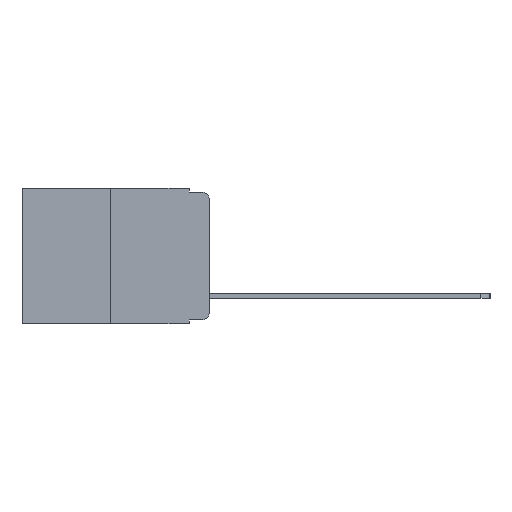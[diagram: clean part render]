
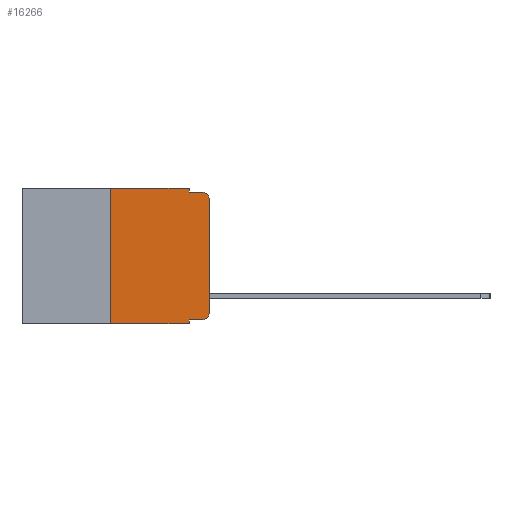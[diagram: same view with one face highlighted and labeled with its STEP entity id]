
A CAD part, left-side view. The second image highlights one B-rep face of the part: STEP entity #16266.
In plain terms, the highlighted planar face has unit normal (-1, 0, 0).
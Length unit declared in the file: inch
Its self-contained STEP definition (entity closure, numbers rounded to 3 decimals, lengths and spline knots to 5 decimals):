
#207 = CARTESIAN_POINT ( 'NONE',  ( 0., 0.051, -0.333 ) ) ;
#868 = ORIENTED_EDGE ( 'NONE', *, *, #16765, .T. ) ;
#1029 = DIRECTION ( 'NONE',  ( -1., 0., 0. ) ) ;
#1169 = CARTESIAN_POINT ( 'NONE',  ( 0., 0., -0.03 ) ) ;
#1591 = VECTOR ( 'NONE', #9328, 39.37008 ) ;
#1666 = VERTEX_POINT ( 'NONE', #6578 ) ;
#1688 = ORIENTED_EDGE ( 'NONE', *, *, #2885, .T. ) ;
#2386 = LINE ( 'NONE', #5557, #13495 ) ;
#2468 = EDGE_LOOP ( 'NONE', ( #868, #10151, #3835, #2747, #3150, #14871, #12457, #14126, #10528, #1688 ) ) ;
#2552 = DIRECTION ( 'NONE',  ( 0., -1., 0. ) ) ;
#2593 = CARTESIAN_POINT ( 'NONE',  ( 0., 0.051, 0. ) ) ;
#2747 = ORIENTED_EDGE ( 'NONE', *, *, #11680, .F. ) ;
#2823 = CIRCLE ( 'NONE', #15723, 0.02 ) ;
#2885 = EDGE_CURVE ( 'NONE', #5201, #4360, #8618, .T. ) ;
#2953 = VERTEX_POINT ( 'NONE', #6489 ) ;
#3044 = AXIS2_PLACEMENT_3D ( 'NONE', #14238, #14297, #5747 ) ;
#3091 = DIRECTION ( 'NONE',  ( 0., 0., -1. ) ) ;
#3150 = ORIENTED_EDGE ( 'NONE', *, *, #5039, .F. ) ;
#3338 = LINE ( 'NONE', #12954, #6807 ) ;
#3835 = ORIENTED_EDGE ( 'NONE', *, *, #14024, .F. ) ;
#3936 = CARTESIAN_POINT ( 'NONE',  ( 0., 0., 0. ) ) ;
#4185 = LINE ( 'NONE', #10406, #15568 ) ;
#4239 = VERTEX_POINT ( 'NONE', #1169 ) ;
#4281 = PLANE ( 'NONE',  #3044 ) ;
#4360 = VERTEX_POINT ( 'NONE', #13071 ) ;
#4916 = VECTOR ( 'NONE', #13665, 39.37008 ) ;
#5039 = EDGE_CURVE ( 'NONE', #15946, #13731, #14305, .T. ) ;
#5201 = VERTEX_POINT ( 'NONE', #18048 ) ;
#5278 = CARTESIAN_POINT ( 'NONE',  ( 0., 0.02, -0.313 ) ) ;
#5400 = DIRECTION ( 'NONE',  ( 0., 0., 1. ) ) ;
#5557 = CARTESIAN_POINT ( 'NONE',  ( 0., 0.25, 0. ) ) ;
#5747 = DIRECTION ( 'NONE',  ( 0., 0., -1. ) ) ;
#6213 = VERTEX_POINT ( 'NONE', #15892 ) ;
#6386 = CARTESIAN_POINT ( 'NONE',  ( 0., 0.051, -0.01 ) ) ;
#6414 = CARTESIAN_POINT ( 'NONE',  ( 0., 0.473, -0.343 ) ) ;
#6489 = CARTESIAN_POINT ( 'NONE',  ( 0., 0.051, -0.343 ) ) ;
#6578 = CARTESIAN_POINT ( 'NONE',  ( 0., 0.02, -0.01 ) ) ;
#6728 = VECTOR ( 'NONE', #9262, 39.37008 ) ;
#6807 = VECTOR ( 'NONE', #10155, 39.37008 ) ;
#7189 = DIRECTION ( 'NONE',  ( -1., 0., 0. ) ) ;
#7321 = VECTOR ( 'NONE', #5400, 39.37008 ) ;
#7335 = EDGE_CURVE ( 'NONE', #11164, #5201, #15404, .T. ) ;
#7888 = VECTOR ( 'NONE', #2552, 39.37008 ) ;
#8353 = EDGE_CURVE ( 'NONE', #6213, #2953, #9427, .T. ) ;
#8431 = DIRECTION ( 'NONE',  ( 0., 0., 1. ) ) ;
#8618 = CIRCLE ( 'NONE', #9480, 0.02 ) ;
#8851 = EDGE_CURVE ( 'NONE', #11164, #2953, #4185, .T. ) ;
#9262 = DIRECTION ( 'NONE',  ( 0., -1., 0. ) ) ;
#9328 = DIRECTION ( 'NONE',  ( 0., -1., 0. ) ) ;
#9427 = LINE ( 'NONE', #6414, #1591 ) ;
#9480 = AXIS2_PLACEMENT_3D ( 'NONE', #5278, #1029, #14162 ) ;
#9791 = CARTESIAN_POINT ( 'NONE',  ( 0., 0.051, -0.333 ) ) ;
#10151 = ORIENTED_EDGE ( 'NONE', *, *, #12604, .T. ) ;
#10155 = DIRECTION ( 'NONE',  ( 0., 0., -1. ) ) ;
#10406 = CARTESIAN_POINT ( 'NONE',  ( 0., 0.051, 0. ) ) ;
#10528 = ORIENTED_EDGE ( 'NONE', *, *, #7335, .T. ) ;
#11105 = LINE ( 'NONE', #3936, #7321 ) ;
#11164 = VERTEX_POINT ( 'NONE', #207 ) ;
#11286 = VERTEX_POINT ( 'NONE', #6386 ) ;
#11680 = EDGE_CURVE ( 'NONE', #13731, #11286, #3338, .T. ) ;
#12094 = CARTESIAN_POINT ( 'NONE',  ( 0., 0.25, 0. ) ) ;
#12166 = CARTESIAN_POINT ( 'NONE',  ( 0., 0.473, 0. ) ) ;
#12238 = CARTESIAN_POINT ( 'NONE',  ( 0., 0.051, -0.01 ) ) ;
#12457 = ORIENTED_EDGE ( 'NONE', *, *, #8353, .T. ) ;
#12582 = LINE ( 'NONE', #12238, #4916 ) ;
#12604 = EDGE_CURVE ( 'NONE', #4239, #1666, #2823, .T. ) ;
#12954 = CARTESIAN_POINT ( 'NONE',  ( 0., 0.051, 0. ) ) ;
#13071 = CARTESIAN_POINT ( 'NONE',  ( 0., 0., -0.313 ) ) ;
#13118 = EDGE_CURVE ( 'NONE', #6213, #15946, #2386, .T. ) ;
#13495 = VECTOR ( 'NONE', #8431, 39.37008 ) ;
#13665 = DIRECTION ( 'NONE',  ( 0., -1., 0. ) ) ;
#13731 = VERTEX_POINT ( 'NONE', #2593 ) ;
#14024 = EDGE_CURVE ( 'NONE', #11286, #1666, #12582, .T. ) ;
#14126 = ORIENTED_EDGE ( 'NONE', *, *, #8851, .F. ) ;
#14162 = DIRECTION ( 'NONE',  ( 0., 0., -1. ) ) ;
#14238 = CARTESIAN_POINT ( 'NONE',  ( 0., 0.473, 0. ) ) ;
#14297 = DIRECTION ( 'NONE',  ( 1., 0., 0. ) ) ;
#14305 = LINE ( 'NONE', #12166, #6728 ) ;
#14871 = ORIENTED_EDGE ( 'NONE', *, *, #13118, .F. ) ;
#15404 = LINE ( 'NONE', #9791, #7888 ) ;
#15568 = VECTOR ( 'NONE', #3091, 39.37008 ) ;
#15640 = CARTESIAN_POINT ( 'NONE',  ( 0., 0.02, -0.03 ) ) ;
#15723 = AXIS2_PLACEMENT_3D ( 'NONE', #15640, #7189, #17032 ) ;
#15892 = CARTESIAN_POINT ( 'NONE',  ( 0., 0.25, -0.343 ) ) ;
#15946 = VERTEX_POINT ( 'NONE', #12094 ) ;
#16266 = ADVANCED_FACE ( 'NONE', ( #17036 ), #4281, .F. ) ;
#16765 = EDGE_CURVE ( 'NONE', #4360, #4239, #11105, .T. ) ;
#17032 = DIRECTION ( 'NONE',  ( 0., 0., -1. ) ) ;
#17036 = FACE_OUTER_BOUND ( 'NONE', #2468, .T. ) ;
#18048 = CARTESIAN_POINT ( 'NONE',  ( 0., 0.02, -0.333 ) ) ;
